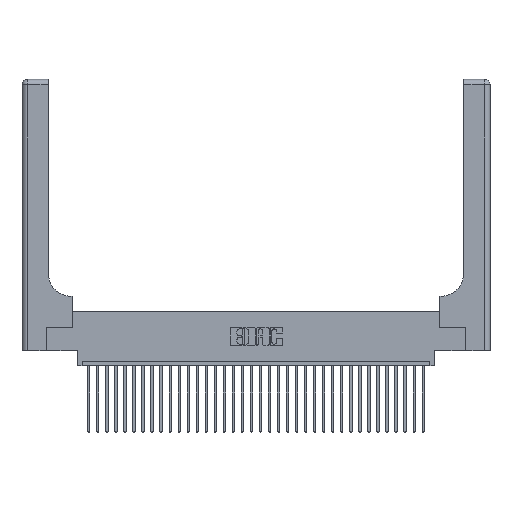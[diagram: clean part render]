
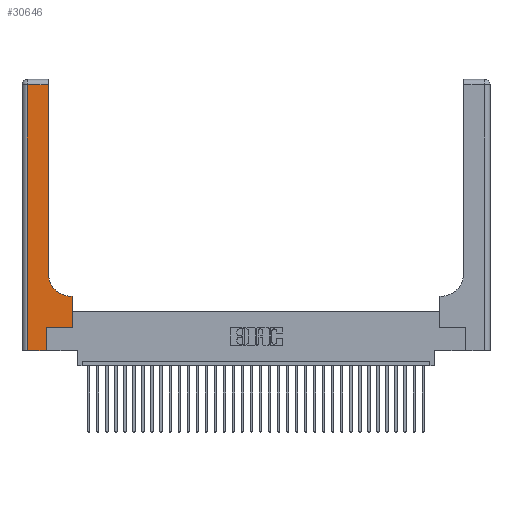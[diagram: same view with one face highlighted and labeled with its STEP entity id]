
A CAD part, top view. The second image highlights one B-rep face of the part: STEP entity #30646.
In plain terms, the highlighted planar face has unit normal (0, 0, 1).
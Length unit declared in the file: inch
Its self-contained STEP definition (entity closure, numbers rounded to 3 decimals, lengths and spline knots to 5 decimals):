
#761 = VECTOR ( 'NONE', #26724, 39.37008 ) ;
#892 = CARTESIAN_POINT ( 'NONE',  ( 0.269, 0.25, 0.37 ) ) ;
#1073 = EDGE_CURVE ( 'NONE', #11943, #8867, #8509, .T. ) ;
#1109 = CARTESIAN_POINT ( 'NONE',  ( 0.269, 0., 0.37 ) ) ;
#2089 = EDGE_CURVE ( 'NONE', #24567, #28946, #10908, .T. ) ;
#2365 = VERTEX_POINT ( 'NONE', #4168 ) ;
#2717 = ORIENTED_EDGE ( 'NONE', *, *, #15245, .T. ) ;
#3334 = LINE ( 'NONE', #11860, #9642 ) ;
#3870 = ORIENTED_EDGE ( 'NONE', *, *, #2089, .T. ) ;
#4168 = CARTESIAN_POINT ( 'NONE',  ( 0.06, 0., 0.37 ) ) ;
#4970 = ORIENTED_EDGE ( 'NONE', *, *, #5882, .T. ) ;
#5612 = VECTOR ( 'NONE', #28898, 39.37008 ) ;
#5882 = EDGE_CURVE ( 'NONE', #8867, #13283, #20042, .T. ) ;
#6061 = FACE_OUTER_BOUND ( 'NONE', #12482, .T. ) ;
#6270 = LINE ( 'NONE', #32649, #33365 ) ;
#6448 = CARTESIAN_POINT ( 'NONE',  ( 0.2915, 0.85, 0.37 ) ) ;
#7522 = ORIENTED_EDGE ( 'NONE', *, *, #32932, .T. ) ;
#7894 = ORIENTED_EDGE ( 'NONE', *, *, #27648, .T. ) ;
#8288 = DIRECTION ( 'NONE',  ( 1., 0., 0. ) ) ;
#8509 = LINE ( 'NONE', #28453, #16796 ) ;
#8768 = CARTESIAN_POINT ( 'NONE',  ( 0., 3., 0.37 ) ) ;
#8867 = VERTEX_POINT ( 'NONE', #17323 ) ;
#8868 = CARTESIAN_POINT ( 'NONE',  ( 0.269, 0., 0.37 ) ) ;
#9504 = CARTESIAN_POINT ( 'NONE',  ( 0., 2.94, 0.37 ) ) ;
#9642 = VECTOR ( 'NONE', #30457, 39.37008 ) ;
#10760 = CARTESIAN_POINT ( 'NONE',  ( 0.06, 3., 0.37 ) ) ;
#10908 = LINE ( 'NONE', #8868, #17950 ) ;
#10992 = DIRECTION ( 'NONE',  ( 0., 0., -1. ) ) ;
#11116 = EDGE_CURVE ( 'NONE', #25471, #2365, #24981, .T. ) ;
#11342 = DIRECTION ( 'NONE',  ( -1., 0., 0. ) ) ;
#11788 = CARTESIAN_POINT ( 'NONE',  ( 0.5585, 0.25, 0.37 ) ) ;
#11859 = LINE ( 'NONE', #18633, #5612 ) ;
#11860 = CARTESIAN_POINT ( 'NONE',  ( 0.269, 0.25, 0.37 ) ) ;
#11887 = CARTESIAN_POINT ( 'NONE',  ( 0.5585, 0.6, 0.37 ) ) ;
#11894 = VERTEX_POINT ( 'NONE', #25007 ) ;
#11943 = VERTEX_POINT ( 'NONE', #11887 ) ;
#12482 = EDGE_LOOP ( 'NONE', ( #2717, #7522, #30697, #7894, #3870, #32676, #30524, #31571, #4970 ) ) ;
#12550 = DIRECTION ( 'NONE',  ( -1., 0., 0. ) ) ;
#13283 = VERTEX_POINT ( 'NONE', #6448 ) ;
#13494 = VERTEX_POINT ( 'NONE', #11788 ) ;
#13527 = AXIS2_PLACEMENT_3D ( 'NONE', #18831, #16268, #8288 ) ;
#13805 = VECTOR ( 'NONE', #14821, 39.37008 ) ;
#14248 = DIRECTION ( 'NONE',  ( 0., 1., 0. ) ) ;
#14821 = DIRECTION ( 'NONE',  ( -1., 0., 0. ) ) ;
#15245 = EDGE_CURVE ( 'NONE', #13283, #11894, #6270, .T. ) ;
#16268 = DIRECTION ( 'NONE',  ( 0., 0., -1. ) ) ;
#16698 = LINE ( 'NONE', #9504, #13805 ) ;
#16796 = VECTOR ( 'NONE', #12550, 39.37008 ) ;
#17323 = CARTESIAN_POINT ( 'NONE',  ( 0.5415, 0.6, 0.37 ) ) ;
#17950 = VECTOR ( 'NONE', #27539, 39.37008 ) ;
#18633 = CARTESIAN_POINT ( 'NONE',  ( 0., 0., 0.37 ) ) ;
#18831 = CARTESIAN_POINT ( 'NONE',  ( 0.5415, 0.85, 0.37 ) ) ;
#20042 = CIRCLE ( 'NONE', #13527, 0.25 ) ;
#21171 = LINE ( 'NONE', #34456, #761 ) ;
#22478 = VECTOR ( 'NONE', #28975, 39.37008 ) ;
#23534 = EDGE_CURVE ( 'NONE', #28946, #13494, #3334, .T. ) ;
#24292 = PLANE ( 'NONE',  #30477 ) ;
#24567 = VERTEX_POINT ( 'NONE', #1109 ) ;
#24981 = LINE ( 'NONE', #10760, #22478 ) ;
#25007 = CARTESIAN_POINT ( 'NONE',  ( 0.2915, 2.94, 0.37 ) ) ;
#25471 = VERTEX_POINT ( 'NONE', #31669 ) ;
#26724 = DIRECTION ( 'NONE',  ( 0., 1., 0. ) ) ;
#27539 = DIRECTION ( 'NONE',  ( 0., 1., 0. ) ) ;
#27648 = EDGE_CURVE ( 'NONE', #2365, #24567, #11859, .T. ) ;
#28352 = EDGE_CURVE ( 'NONE', #13494, #11943, #21171, .T. ) ;
#28453 = CARTESIAN_POINT ( 'NONE',  ( 0.2915, 0.6, 0.37 ) ) ;
#28898 = DIRECTION ( 'NONE',  ( 1., 0., 0. ) ) ;
#28946 = VERTEX_POINT ( 'NONE', #892 ) ;
#28975 = DIRECTION ( 'NONE',  ( 0., -1., 0. ) ) ;
#30457 = DIRECTION ( 'NONE',  ( 1., 0., 0. ) ) ;
#30477 = AXIS2_PLACEMENT_3D ( 'NONE', #8768, #10992, #11342 ) ;
#30524 = ORIENTED_EDGE ( 'NONE', *, *, #28352, .T. ) ;
#30646 = ADVANCED_FACE ( 'NONE', ( #6061 ), #24292, .F. ) ;
#30697 = ORIENTED_EDGE ( 'NONE', *, *, #11116, .T. ) ;
#31571 = ORIENTED_EDGE ( 'NONE', *, *, #1073, .T. ) ;
#31669 = CARTESIAN_POINT ( 'NONE',  ( 0.06, 2.94, 0.37 ) ) ;
#32649 = CARTESIAN_POINT ( 'NONE',  ( 0.2915, 3., 0.37 ) ) ;
#32676 = ORIENTED_EDGE ( 'NONE', *, *, #23534, .T. ) ;
#32932 = EDGE_CURVE ( 'NONE', #11894, #25471, #16698, .T. ) ;
#33365 = VECTOR ( 'NONE', #14248, 39.37008 ) ;
#34456 = CARTESIAN_POINT ( 'NONE',  ( 0.5585, 0.25, 0.37 ) ) ;
